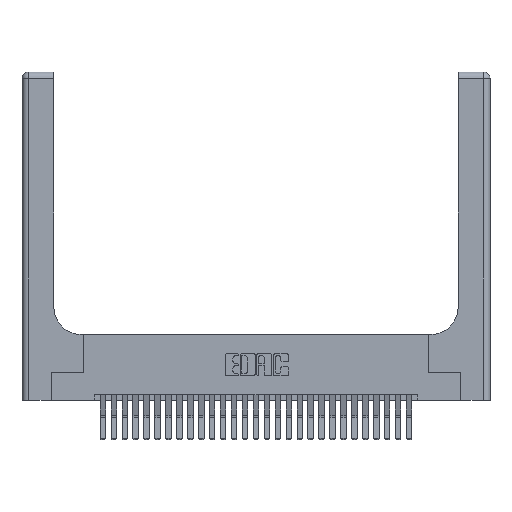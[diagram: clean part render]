
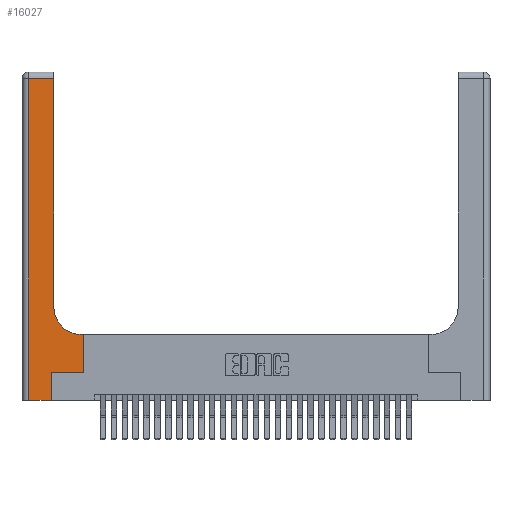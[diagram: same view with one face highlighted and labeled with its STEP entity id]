
A CAD part, top view. The second image highlights one B-rep face of the part: STEP entity #16027.
In plain terms, the highlighted planar face has unit normal (0, 0, 1).
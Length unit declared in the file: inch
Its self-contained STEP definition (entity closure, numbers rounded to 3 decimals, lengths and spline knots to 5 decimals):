
#19 = CARTESIAN_POINT ( 'NONE',  ( 0.06, 2.94, 0.37 ) ) ;
#539 = VECTOR ( 'NONE', #11750, 39.37008 ) ;
#737 = LINE ( 'NONE', #18682, #14064 ) ;
#752 = DIRECTION ( 'NONE',  ( 0., -1., 0. ) ) ;
#837 = LINE ( 'NONE', #9237, #24590 ) ;
#986 = DIRECTION ( 'NONE',  ( 1., 0., 0. ) ) ;
#1452 = EDGE_CURVE ( 'NONE', #9608, #7491, #8470, .T. ) ;
#2517 = ORIENTED_EDGE ( 'NONE', *, *, #24219, .T. ) ;
#2940 = CARTESIAN_POINT ( 'NONE',  ( 0.5415, 0.6, 0.37 ) ) ;
#3020 = VERTEX_POINT ( 'NONE', #10079 ) ;
#4358 = ORIENTED_EDGE ( 'NONE', *, *, #20662, .T. ) ;
#4563 = CARTESIAN_POINT ( 'NONE',  ( 0., 3., 0.37 ) ) ;
#4983 = LINE ( 'NONE', #13087, #25176 ) ;
#5051 = ORIENTED_EDGE ( 'NONE', *, *, #13424, .T. ) ;
#5423 = VECTOR ( 'NONE', #18356, 39.37008 ) ;
#5533 = ORIENTED_EDGE ( 'NONE', *, *, #19530, .T. ) ;
#5916 = CARTESIAN_POINT ( 'NONE',  ( 0.269, 0., 0.37 ) ) ;
#6306 = DIRECTION ( 'NONE',  ( 0., 0., -1. ) ) ;
#6428 = VERTEX_POINT ( 'NONE', #2940 ) ;
#7458 = VERTEX_POINT ( 'NONE', #8583 ) ;
#7491 = VERTEX_POINT ( 'NONE', #8283 ) ;
#8270 = ORIENTED_EDGE ( 'NONE', *, *, #1452, .T. ) ;
#8283 = CARTESIAN_POINT ( 'NONE',  ( 0.5585, 0.25, 0.37 ) ) ;
#8349 = VECTOR ( 'NONE', #19534, 39.37008 ) ;
#8470 = LINE ( 'NONE', #9748, #26774 ) ;
#8583 = CARTESIAN_POINT ( 'NONE',  ( 0.2915, 0.85, 0.37 ) ) ;
#9237 = CARTESIAN_POINT ( 'NONE',  ( 0.2915, 3., 0.37 ) ) ;
#9337 = CARTESIAN_POINT ( 'NONE',  ( 0., 2.94, 0.37 ) ) ;
#9465 = CARTESIAN_POINT ( 'NONE',  ( 0.269, 0.25, 0.37 ) ) ;
#9608 = VERTEX_POINT ( 'NONE', #9465 ) ;
#9748 = CARTESIAN_POINT ( 'NONE',  ( 0.269, 0.25, 0.37 ) ) ;
#10079 = CARTESIAN_POINT ( 'NONE',  ( 0.2915, 2.94, 0.37 ) ) ;
#10500 = AXIS2_PLACEMENT_3D ( 'NONE', #4563, #17862, #29205 ) ;
#10862 = LINE ( 'NONE', #5916, #8349 ) ;
#11620 = CARTESIAN_POINT ( 'NONE',  ( 0.06, 0., 0.37 ) ) ;
#11740 = PLANE ( 'NONE',  #10500 ) ;
#11741 = DIRECTION ( 'NONE',  ( 0., 1., 0. ) ) ;
#11750 = DIRECTION ( 'NONE',  ( -1., 0., 0. ) ) ;
#12524 = ORIENTED_EDGE ( 'NONE', *, *, #27015, .T. ) ;
#13087 = CARTESIAN_POINT ( 'NONE',  ( 0.5585, 0.25, 0.37 ) ) ;
#13238 = CIRCLE ( 'NONE', #22229, 0.25 ) ;
#13424 = EDGE_CURVE ( 'NONE', #28057, #24350, #737, .T. ) ;
#13531 = ORIENTED_EDGE ( 'NONE', *, *, #24881, .T. ) ;
#14064 = VECTOR ( 'NONE', #752, 39.37008 ) ;
#14386 = EDGE_CURVE ( 'NONE', #24350, #25243, #17767, .T. ) ;
#14861 = CARTESIAN_POINT ( 'NONE',  ( 0.269, 0., 0.37 ) ) ;
#15357 = ORIENTED_EDGE ( 'NONE', *, *, #21536, .T. ) ;
#16027 = ADVANCED_FACE ( 'NONE', ( #24759 ), #11740, .F. ) ;
#16109 = CARTESIAN_POINT ( 'NONE',  ( 0.5585, 0.6, 0.37 ) ) ;
#17767 = LINE ( 'NONE', #27658, #5423 ) ;
#17862 = DIRECTION ( 'NONE',  ( 0., 0., -1. ) ) ;
#18356 = DIRECTION ( 'NONE',  ( 1., 0., 0. ) ) ;
#18682 = CARTESIAN_POINT ( 'NONE',  ( 0.06, 3., 0.37 ) ) ;
#18859 = VERTEX_POINT ( 'NONE', #16109 ) ;
#19530 = EDGE_CURVE ( 'NONE', #7458, #3020, #837, .T. ) ;
#19534 = DIRECTION ( 'NONE',  ( 0., 1., 0. ) ) ;
#20117 = CARTESIAN_POINT ( 'NONE',  ( 0.5415, 0.85, 0.37 ) ) ;
#20185 = EDGE_LOOP ( 'NONE', ( #5533, #15357, #5051, #23694, #4358, #8270, #13531, #2517, #12524 ) ) ;
#20538 = VECTOR ( 'NONE', #27250, 39.37008 ) ;
#20662 = EDGE_CURVE ( 'NONE', #25243, #9608, #10862, .T. ) ;
#21536 = EDGE_CURVE ( 'NONE', #3020, #28057, #26803, .T. ) ;
#22229 = AXIS2_PLACEMENT_3D ( 'NONE', #20117, #6306, #22400 ) ;
#22400 = DIRECTION ( 'NONE',  ( 1., 0., 0. ) ) ;
#23694 = ORIENTED_EDGE ( 'NONE', *, *, #14386, .T. ) ;
#24219 = EDGE_CURVE ( 'NONE', #18859, #6428, #27356, .T. ) ;
#24350 = VERTEX_POINT ( 'NONE', #11620 ) ;
#24590 = VECTOR ( 'NONE', #27179, 39.37008 ) ;
#24759 = FACE_OUTER_BOUND ( 'NONE', #20185, .T. ) ;
#24881 = EDGE_CURVE ( 'NONE', #7491, #18859, #4983, .T. ) ;
#25176 = VECTOR ( 'NONE', #11741, 39.37008 ) ;
#25243 = VERTEX_POINT ( 'NONE', #14861 ) ;
#26774 = VECTOR ( 'NONE', #986, 39.37008 ) ;
#26803 = LINE ( 'NONE', #9337, #539 ) ;
#27015 = EDGE_CURVE ( 'NONE', #6428, #7458, #13238, .T. ) ;
#27042 = CARTESIAN_POINT ( 'NONE',  ( 0.2915, 0.6, 0.37 ) ) ;
#27179 = DIRECTION ( 'NONE',  ( 0., 1., 0. ) ) ;
#27250 = DIRECTION ( 'NONE',  ( -1., 0., 0. ) ) ;
#27356 = LINE ( 'NONE', #27042, #20538 ) ;
#27658 = CARTESIAN_POINT ( 'NONE',  ( 0., 0., 0.37 ) ) ;
#28057 = VERTEX_POINT ( 'NONE', #19 ) ;
#29205 = DIRECTION ( 'NONE',  ( -1., 0., 0. ) ) ;
